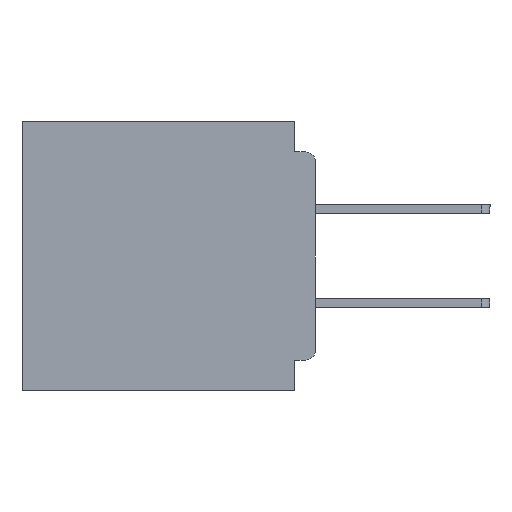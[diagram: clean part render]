
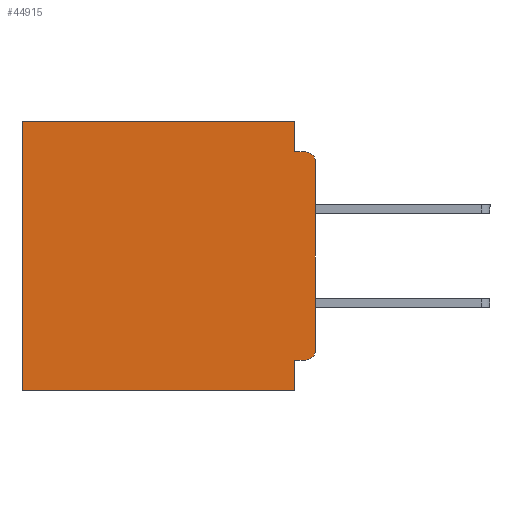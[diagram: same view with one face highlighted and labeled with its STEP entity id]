
A CAD part, left-side view. The second image highlights one B-rep face of the part: STEP entity #44915.
In plain terms, the highlighted planar face has unit normal (-1, 0, 0).
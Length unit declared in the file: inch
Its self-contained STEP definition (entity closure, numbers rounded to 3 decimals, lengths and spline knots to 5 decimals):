
#1648 = EDGE_CURVE ( 'NONE', #41967, #51165, #49549, .T. ) ;
#2080 = CARTESIAN_POINT ( 'NONE',  ( 0.3, 0., 0. ) ) ;
#2170 = VECTOR ( 'NONE', #36166, 39.37008 ) ;
#3664 = ORIENTED_EDGE ( 'NONE', *, *, #21251, .F. ) ;
#3716 = CARTESIAN_POINT ( 'NONE',  ( 0.3, 0., -0.4 ) ) ;
#3923 = ORIENTED_EDGE ( 'NONE', *, *, #23032, .F. ) ;
#4776 = CARTESIAN_POINT ( 'NONE',  ( 0.3, 0.015, -0.355 ) ) ;
#5858 = EDGE_CURVE ( 'NONE', #53500, #51165, #35235, .T. ) ;
#6525 = EDGE_CURVE ( 'NONE', #55325, #42957, #11613, .T. ) ;
#7038 = CIRCLE ( 'NONE', #27317, 0.015 ) ;
#7431 = EDGE_CURVE ( 'NONE', #31269, #42957, #14262, .T. ) ;
#8539 = ORIENTED_EDGE ( 'NONE', *, *, #26062, .F. ) ;
#8606 = CARTESIAN_POINT ( 'NONE',  ( 0.3, 0.031, -0.355 ) ) ;
#9111 = CARTESIAN_POINT ( 'NONE',  ( 0.3, 0., -0.4 ) ) ;
#9130 = CARTESIAN_POINT ( 'NONE',  ( 0.3, 0.437, -0.4 ) ) ;
#10711 = DIRECTION ( 'NONE',  ( -1., 0., 0. ) ) ;
#10955 = ORIENTED_EDGE ( 'NONE', *, *, #7431, .T. ) ;
#11613 = LINE ( 'NONE', #3716, #22365 ) ;
#11770 = VERTEX_POINT ( 'NONE', #4776 ) ;
#12154 = CARTESIAN_POINT ( 'NONE',  ( 0.3, 0.031, -0.4 ) ) ;
#13182 = VECTOR ( 'NONE', #29858, 39.37008 ) ;
#13730 = LINE ( 'NONE', #52732, #50098 ) ;
#14262 = LINE ( 'NONE', #56319, #27793 ) ;
#17268 = DIRECTION ( 'NONE',  ( -1., 0., 0. ) ) ;
#17340 = VECTOR ( 'NONE', #29765, 39.37008 ) ;
#21251 = EDGE_CURVE ( 'NONE', #11770, #54837, #13730, .T. ) ;
#22365 = VECTOR ( 'NONE', #31083, 39.37008 ) ;
#23032 = EDGE_CURVE ( 'NONE', #54837, #55325, #24052, .T. ) ;
#24052 = LINE ( 'NONE', #47287, #45419 ) ;
#24446 = DIRECTION ( 'NONE',  ( 0., 0., -1. ) ) ;
#24941 = ORIENTED_EDGE ( 'NONE', *, *, #5858, .T. ) ;
#25360 = CARTESIAN_POINT ( 'NONE',  ( 0.3, 0., -0.06 ) ) ;
#25368 = CARTESIAN_POINT ( 'NONE',  ( 0.3, 0.031, -0.045 ) ) ;
#25884 = CARTESIAN_POINT ( 'NONE',  ( 0.3, 0., -0.045 ) ) ;
#26062 = EDGE_CURVE ( 'NONE', #57761, #41967, #38592, .T. ) ;
#27317 = AXIS2_PLACEMENT_3D ( 'NONE', #38006, #10711, #42608 ) ;
#27466 = DIRECTION ( 'NONE',  ( 0., 0., -1. ) ) ;
#27793 = VECTOR ( 'NONE', #24446, 39.37008 ) ;
#29461 = ORIENTED_EDGE ( 'NONE', *, *, #57220, .T. ) ;
#29765 = DIRECTION ( 'NONE',  ( 0., 0., -1. ) ) ;
#29858 = DIRECTION ( 'NONE',  ( 0., -1., 0. ) ) ;
#30634 = ORIENTED_EDGE ( 'NONE', *, *, #6525, .F. ) ;
#31083 = DIRECTION ( 'NONE',  ( 0., 1., 0. ) ) ;
#31269 = VERTEX_POINT ( 'NONE', #40307 ) ;
#32115 = AXIS2_PLACEMENT_3D ( 'NONE', #9111, #54799, #27466 ) ;
#34023 = DIRECTION ( 'NONE',  ( 0., 1., 0. ) ) ;
#34613 = CARTESIAN_POINT ( 'NONE',  ( 0.3, 0., -0.34 ) ) ;
#35235 = CIRCLE ( 'NONE', #55353, 0.015 ) ;
#36166 = DIRECTION ( 'NONE',  ( 0., 0., -1. ) ) ;
#38006 = CARTESIAN_POINT ( 'NONE',  ( 0.3, 0.015, -0.34 ) ) ;
#38592 = LINE ( 'NONE', #58911, #2170 ) ;
#38947 = DIRECTION ( 'NONE',  ( 0., 1., 0. ) ) ;
#40258 = VECTOR ( 'NONE', #34023, 39.37008 ) ;
#40307 = CARTESIAN_POINT ( 'NONE',  ( 0.3, 0.437, 0. ) ) ;
#40452 = FACE_OUTER_BOUND ( 'NONE', #46035, .T. ) ;
#41439 = EDGE_CURVE ( 'NONE', #53500, #43324, #53690, .T. ) ;
#41686 = LINE ( 'NONE', #2080, #40258 ) ;
#41967 = VERTEX_POINT ( 'NONE', #25368 ) ;
#42608 = DIRECTION ( 'NONE',  ( 0., 0., -1. ) ) ;
#42957 = VERTEX_POINT ( 'NONE', #9130 ) ;
#43155 = CARTESIAN_POINT ( 'NONE',  ( 0.3, 0., -0.4 ) ) ;
#43324 = VERTEX_POINT ( 'NONE', #34613 ) ;
#43384 = ORIENTED_EDGE ( 'NONE', *, *, #59029, .T. ) ;
#43426 = ORIENTED_EDGE ( 'NONE', *, *, #1648, .F. ) ;
#44538 = CARTESIAN_POINT ( 'NONE',  ( 0.3, 0.015, -0.06 ) ) ;
#44915 = ADVANCED_FACE ( 'NONE', ( #40452 ), #50193, .F. ) ;
#45419 = VECTOR ( 'NONE', #51882, 39.37008 ) ;
#46035 = EDGE_LOOP ( 'NONE', ( #48675, #24941, #43426, #8539, #29461, #10955, #30634, #3923, #3664, #43384 ) ) ;
#47287 = CARTESIAN_POINT ( 'NONE',  ( 0.3, 0.031, -0.4 ) ) ;
#48675 = ORIENTED_EDGE ( 'NONE', *, *, #41439, .F. ) ;
#49101 = DIRECTION ( 'NONE',  ( 0., 0., -1. ) ) ;
#49304 = CARTESIAN_POINT ( 'NONE',  ( 0.3, 0.015, -0.045 ) ) ;
#49549 = LINE ( 'NONE', #25884, #13182 ) ;
#50098 = VECTOR ( 'NONE', #38947, 39.37008 ) ;
#50193 = PLANE ( 'NONE',  #32115 ) ;
#51165 = VERTEX_POINT ( 'NONE', #49304 ) ;
#51882 = DIRECTION ( 'NONE',  ( 0., 0., -1. ) ) ;
#52732 = CARTESIAN_POINT ( 'NONE',  ( 0.3, 0., -0.355 ) ) ;
#53500 = VERTEX_POINT ( 'NONE', #25360 ) ;
#53690 = LINE ( 'NONE', #43155, #17340 ) ;
#54799 = DIRECTION ( 'NONE',  ( 1., 0., 0. ) ) ;
#54837 = VERTEX_POINT ( 'NONE', #8606 ) ;
#55325 = VERTEX_POINT ( 'NONE', #12154 ) ;
#55353 = AXIS2_PLACEMENT_3D ( 'NONE', #44538, #17268, #49101 ) ;
#56105 = CARTESIAN_POINT ( 'NONE',  ( 0.3, 0.031, 0. ) ) ;
#56319 = CARTESIAN_POINT ( 'NONE',  ( 0.3, 0.437, -0.4 ) ) ;
#57220 = EDGE_CURVE ( 'NONE', #57761, #31269, #41686, .T. ) ;
#57761 = VERTEX_POINT ( 'NONE', #56105 ) ;
#58911 = CARTESIAN_POINT ( 'NONE',  ( 0.3, 0.031, 0. ) ) ;
#59029 = EDGE_CURVE ( 'NONE', #11770, #43324, #7038, .T. ) ;
